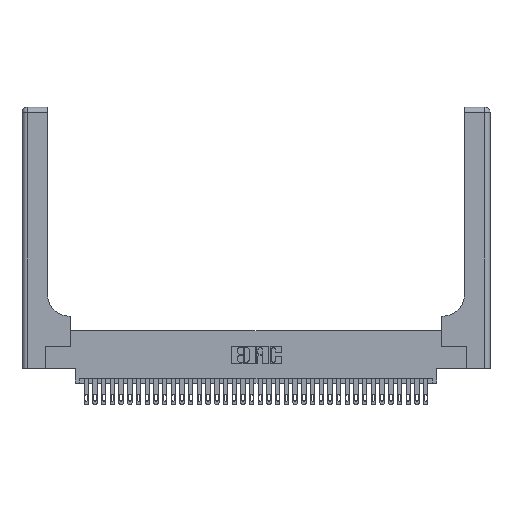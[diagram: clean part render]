
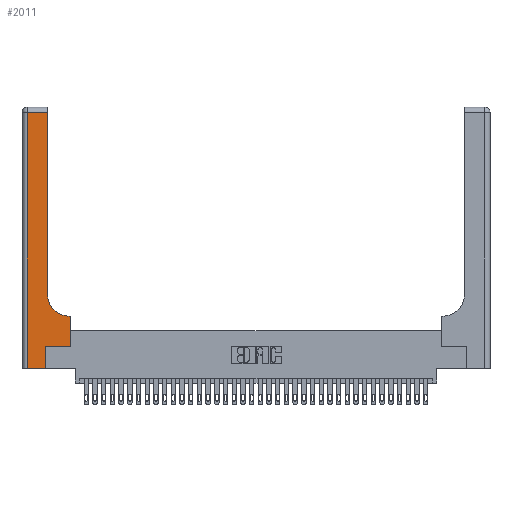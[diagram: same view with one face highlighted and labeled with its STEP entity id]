
A CAD part, top view. The second image highlights one B-rep face of the part: STEP entity #2011.
In plain terms, the highlighted planar face has unit normal (0, 0, 1).
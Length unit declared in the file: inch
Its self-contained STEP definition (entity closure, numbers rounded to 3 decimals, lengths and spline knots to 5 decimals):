
#285 = ORIENTED_EDGE ( 'NONE', *, *, #13726, .T. ) ;
#715 = ORIENTED_EDGE ( 'NONE', *, *, #6657, .T. ) ;
#835 = DIRECTION ( 'NONE',  ( 1., 0., 0. ) ) ;
#1523 = CARTESIAN_POINT ( 'NONE',  ( 0.5585, 0.25, 0.37 ) ) ;
#1912 = VECTOR ( 'NONE', #7038, 39.37008 ) ;
#2011 = ADVANCED_FACE ( 'NONE', ( #33632 ), #12705, .F. ) ;
#2240 = EDGE_CURVE ( 'NONE', #22795, #36031, #34477, .T. ) ;
#2268 = CARTESIAN_POINT ( 'NONE',  ( 0., 0., 0.37 ) ) ;
#4233 = ORIENTED_EDGE ( 'NONE', *, *, #30428, .T. ) ;
#4845 = DIRECTION ( 'NONE',  ( -1., 0., 0. ) ) ;
#4958 = VECTOR ( 'NONE', #10535, 39.37008 ) ;
#5129 = LINE ( 'NONE', #23902, #35393 ) ;
#5255 = CARTESIAN_POINT ( 'NONE',  ( 0.5415, 0.85, 0.37 ) ) ;
#5752 = EDGE_LOOP ( 'NONE', ( #35906, #18652, #26336, #20026, #4233, #285, #7645, #715, #32180 ) ) ;
#6657 = EDGE_CURVE ( 'NONE', #36031, #27758, #28774, .T. ) ;
#7038 = DIRECTION ( 'NONE',  ( 0., 1., 0. ) ) ;
#7645 = ORIENTED_EDGE ( 'NONE', *, *, #2240, .T. ) ;
#7761 = DIRECTION ( 'NONE',  ( 1., 0., 0. ) ) ;
#9753 = EDGE_CURVE ( 'NONE', #28653, #11508, #12484, .T. ) ;
#10378 = DIRECTION ( 'NONE',  ( 0., 0., -1. ) ) ;
#10535 = DIRECTION ( 'NONE',  ( 0., 1., 0. ) ) ;
#10882 = VECTOR ( 'NONE', #835, 39.37008 ) ;
#11508 = VERTEX_POINT ( 'NONE', #21273 ) ;
#12484 = LINE ( 'NONE', #21990, #4958 ) ;
#12657 = EDGE_CURVE ( 'NONE', #11508, #17246, #5129, .T. ) ;
#12705 = PLANE ( 'NONE',  #17063 ) ;
#13726 = EDGE_CURVE ( 'NONE', #32971, #22795, #36697, .T. ) ;
#14247 = CARTESIAN_POINT ( 'NONE',  ( 0.2915, 0.6, 0.37 ) ) ;
#16808 = EDGE_CURVE ( 'NONE', #34920, #26672, #19998, .T. ) ;
#17063 = AXIS2_PLACEMENT_3D ( 'NONE', #18689, #10378, #18553 ) ;
#17246 = VERTEX_POINT ( 'NONE', #36471 ) ;
#18247 = LINE ( 'NONE', #30380, #30319 ) ;
#18399 = CARTESIAN_POINT ( 'NONE',  ( 0.269, 0., 0.37 ) ) ;
#18553 = DIRECTION ( 'NONE',  ( -1., 0., 0. ) ) ;
#18652 = ORIENTED_EDGE ( 'NONE', *, *, #12657, .T. ) ;
#18689 = CARTESIAN_POINT ( 'NONE',  ( 0., 3., 0.37 ) ) ;
#19998 = LINE ( 'NONE', #2268, #35574 ) ;
#20026 = ORIENTED_EDGE ( 'NONE', *, *, #16808, .T. ) ;
#20464 = CARTESIAN_POINT ( 'NONE',  ( 0.5415, 0.6, 0.37 ) ) ;
#20723 = VECTOR ( 'NONE', #35739, 39.37008 ) ;
#20997 = DIRECTION ( 'NONE',  ( 1., 0., 0. ) ) ;
#21273 = CARTESIAN_POINT ( 'NONE',  ( 0.2915, 2.94, 0.37 ) ) ;
#21406 = DIRECTION ( 'NONE',  ( 0., 1., 0. ) ) ;
#21797 = CARTESIAN_POINT ( 'NONE',  ( 0.06, 0., 0.37 ) ) ;
#21822 = CARTESIAN_POINT ( 'NONE',  ( 0.2915, 0.85, 0.37 ) ) ;
#21990 = CARTESIAN_POINT ( 'NONE',  ( 0.2915, 3., 0.37 ) ) ;
#22795 = VERTEX_POINT ( 'NONE', #29726 ) ;
#23040 = CARTESIAN_POINT ( 'NONE',  ( 0.269, 0.25, 0.37 ) ) ;
#23060 = EDGE_CURVE ( 'NONE', #17246, #34920, #35067, .T. ) ;
#23902 = CARTESIAN_POINT ( 'NONE',  ( 0., 2.94, 0.37 ) ) ;
#24259 = DIRECTION ( 'NONE',  ( 0., -1., 0. ) ) ;
#25743 = VECTOR ( 'NONE', #24259, 39.37008 ) ;
#26336 = ORIENTED_EDGE ( 'NONE', *, *, #23060, .T. ) ;
#26644 = CARTESIAN_POINT ( 'NONE',  ( 0.269, 0.25, 0.37 ) ) ;
#26672 = VERTEX_POINT ( 'NONE', #18399 ) ;
#27617 = CARTESIAN_POINT ( 'NONE',  ( 0.06, 3., 0.37 ) ) ;
#27758 = VERTEX_POINT ( 'NONE', #20464 ) ;
#27943 = CIRCLE ( 'NONE', #34752, 0.25 ) ;
#28653 = VERTEX_POINT ( 'NONE', #21822 ) ;
#28774 = LINE ( 'NONE', #14247, #20723 ) ;
#29153 = CARTESIAN_POINT ( 'NONE',  ( 0.5585, 0.6, 0.37 ) ) ;
#29726 = CARTESIAN_POINT ( 'NONE',  ( 0.5585, 0.25, 0.37 ) ) ;
#30319 = VECTOR ( 'NONE', #21406, 39.37008 ) ;
#30380 = CARTESIAN_POINT ( 'NONE',  ( 0.269, 0., 0.37 ) ) ;
#30428 = EDGE_CURVE ( 'NONE', #26672, #32971, #18247, .T. ) ;
#32180 = ORIENTED_EDGE ( 'NONE', *, *, #33179, .T. ) ;
#32971 = VERTEX_POINT ( 'NONE', #26644 ) ;
#33179 = EDGE_CURVE ( 'NONE', #27758, #28653, #27943, .T. ) ;
#33632 = FACE_OUTER_BOUND ( 'NONE', #5752, .T. ) ;
#34477 = LINE ( 'NONE', #1523, #1912 ) ;
#34752 = AXIS2_PLACEMENT_3D ( 'NONE', #5255, #36530, #7761 ) ;
#34920 = VERTEX_POINT ( 'NONE', #21797 ) ;
#35067 = LINE ( 'NONE', #27617, #25743 ) ;
#35393 = VECTOR ( 'NONE', #4845, 39.37008 ) ;
#35574 = VECTOR ( 'NONE', #20997, 39.37008 ) ;
#35739 = DIRECTION ( 'NONE',  ( -1., 0., 0. ) ) ;
#35906 = ORIENTED_EDGE ( 'NONE', *, *, #9753, .T. ) ;
#36031 = VERTEX_POINT ( 'NONE', #29153 ) ;
#36471 = CARTESIAN_POINT ( 'NONE',  ( 0.06, 2.94, 0.37 ) ) ;
#36530 = DIRECTION ( 'NONE',  ( 0., 0., -1. ) ) ;
#36697 = LINE ( 'NONE', #23040, #10882 ) ;
